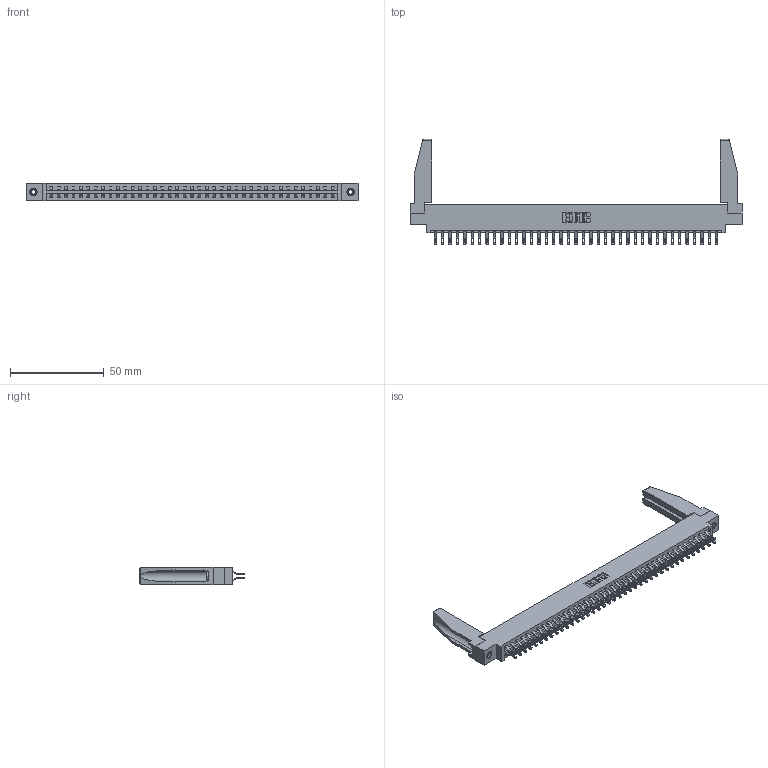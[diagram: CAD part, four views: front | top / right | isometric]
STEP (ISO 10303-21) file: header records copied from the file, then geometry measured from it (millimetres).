
FILE_DESCRIPTION (( 'STEP AP203' ), '1' );
FILE_NAME ('387-078-555-878.STEP', '2019-10-22T06:43:38', ( '' ), ( '' ), 'SwSTEP 2.0', 'SolidWorks 2016', '' );
FILE_SCHEMA (( 'CONFIG_CONTROL_DESIGN' ));
Length unit declared in the file: inch
Products named in the file (5): 345-250-001_345-250-001-102; 345-292-001_555 Tail; 387-078-555-878; 337 Part_0.170 Offset - 0.156 Dia-TI; 307-220-078
Assembly tree (83 placements, depth 2):
  387-078-555-878
    337 Part_0.170 Offset - 0.156 Dia-TI
    345-292-001_555 Tail  x78
    345-250-001_345-250-001-102  x2
    307-220-078  x2
Bounding box: 177.55 x 56.27 x 9.4 mm (x, y, z)
Volume: 22773.3 mm3; surface area: 25992.6 mm2
Topology: 83 solids, 83 shells, 4928 faces, 15395 edges, 10254 vertices
Faces by surface type: plane 2966, cylinder 1946, cone 12, torus 4
Entity records: 33524 total; most frequent: CARTESIAN_POINT 5686, ORIENTED_EDGE 5548, DIRECTION 4818, EDGE_CURVE 2774, VECTOR 2588, LINE 2588, VERTEX_POINT 1844, AXIS2_PLACEMENT_3D 1115
